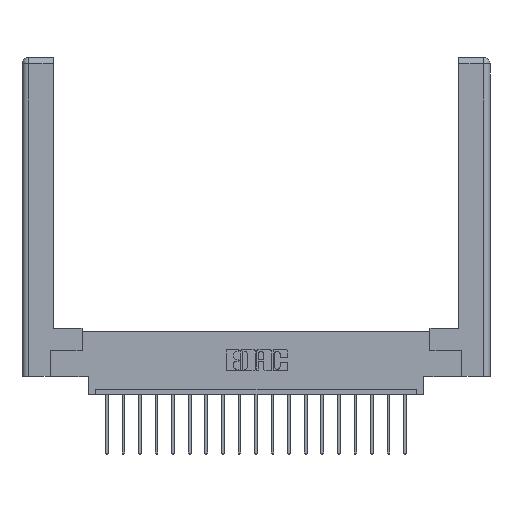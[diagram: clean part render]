
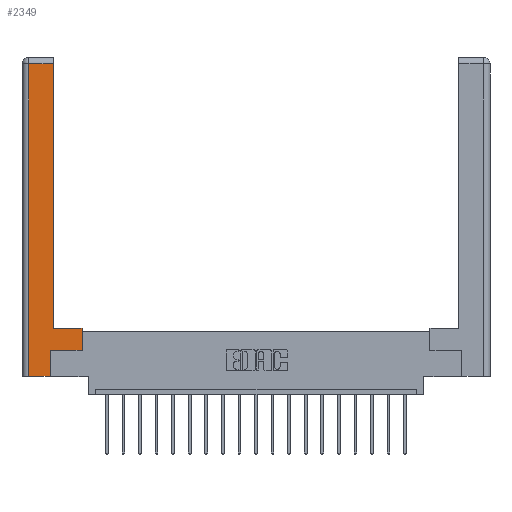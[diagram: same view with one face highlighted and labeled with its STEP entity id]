
A CAD part, top view. The second image highlights one B-rep face of the part: STEP entity #2349.
In plain terms, the highlighted planar face has unit normal (0, 0, 1).
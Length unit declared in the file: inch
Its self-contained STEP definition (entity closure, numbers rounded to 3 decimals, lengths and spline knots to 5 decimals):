
#362 = EDGE_CURVE ( 'NONE', #16933, #14075, #15181, .T. ) ;
#388 = EDGE_CURVE ( 'NONE', #4159, #2547, #11128, .T. ) ;
#723 = EDGE_CURVE ( 'NONE', #13145, #14437, #3665, .T. ) ;
#1186 = LINE ( 'NONE', #17285, #5532 ) ;
#1622 = CARTESIAN_POINT ( 'NONE',  ( 0.565, 0.245, 0. ) ) ;
#2067 = ORIENTED_EDGE ( 'NONE', *, *, #10837, .T. ) ;
#2349 = ADVANCED_FACE ( 'NONE', ( #7881 ), #5505, .F. ) ;
#2424 = VERTEX_POINT ( 'NONE', #3935 ) ;
#2462 = LINE ( 'NONE', #14794, #9640 ) ;
#2547 = VERTEX_POINT ( 'NONE', #1622 ) ;
#3395 = ORIENTED_EDGE ( 'NONE', *, *, #723, .T. ) ;
#3430 = DIRECTION ( 'NONE',  ( 1., 0., 0. ) ) ;
#3432 = VECTOR ( 'NONE', #10427, 39.37008 ) ;
#3541 = DIRECTION ( 'NONE',  ( 0., -1., 0. ) ) ;
#3665 = LINE ( 'NONE', #10676, #6324 ) ;
#3935 = CARTESIAN_POINT ( 'NONE',  ( 0.565, 0.45, 0. ) ) ;
#3956 = ORIENTED_EDGE ( 'NONE', *, *, #388, .T. ) ;
#4159 = VERTEX_POINT ( 'NONE', #4617 ) ;
#4617 = CARTESIAN_POINT ( 'NONE',  ( 0.265, 0.245, 0. ) ) ;
#5131 = DIRECTION ( 'NONE',  ( 1., 0., 0. ) ) ;
#5505 = PLANE ( 'NONE',  #16277 ) ;
#5532 = VECTOR ( 'NONE', #3430, 39.37008 ) ;
#5802 = LINE ( 'NONE', #10413, #13970 ) ;
#6008 = ORIENTED_EDGE ( 'NONE', *, *, #11953, .T. ) ;
#6324 = VECTOR ( 'NONE', #3541, 39.37008 ) ;
#6452 = LINE ( 'NONE', #17853, #6679 ) ;
#6679 = VECTOR ( 'NONE', #18226, 39.37008 ) ;
#6786 = CARTESIAN_POINT ( 'NONE',  ( 0.0615, 0., 0. ) ) ;
#7219 = DIRECTION ( 'NONE',  ( 0., 1., 0. ) ) ;
#7834 = EDGE_LOOP ( 'NONE', ( #15627, #13784, #3395, #6008, #15036, #3956, #2067, #12149 ) ) ;
#7881 = FACE_OUTER_BOUND ( 'NONE', #7834, .T. ) ;
#8752 = EDGE_CURVE ( 'NONE', #2424, #16933, #12839, .T. ) ;
#8883 = VERTEX_POINT ( 'NONE', #18029 ) ;
#9640 = VECTOR ( 'NONE', #7219, 39.37008 ) ;
#9772 = DIRECTION ( 'NONE',  ( -1., 0., 0. ) ) ;
#10413 = CARTESIAN_POINT ( 'NONE',  ( 0.265, 0.245, 0. ) ) ;
#10427 = DIRECTION ( 'NONE',  ( 0., 1., 0. ) ) ;
#10676 = CARTESIAN_POINT ( 'NONE',  ( 0.0615, 0., 0. ) ) ;
#10837 = EDGE_CURVE ( 'NONE', #2547, #2424, #2462, .T. ) ;
#11128 = LINE ( 'NONE', #18882, #19064 ) ;
#11131 = EDGE_CURVE ( 'NONE', #8883, #4159, #5802, .T. ) ;
#11900 = CARTESIAN_POINT ( 'NONE',  ( 0.0615, 2.94, 0. ) ) ;
#11953 = EDGE_CURVE ( 'NONE', #14437, #8883, #1186, .T. ) ;
#12149 = ORIENTED_EDGE ( 'NONE', *, *, #8752, .T. ) ;
#12839 = LINE ( 'NONE', #17646, #18861 ) ;
#12863 = DIRECTION ( 'NONE',  ( 0., 0., -1. ) ) ;
#13145 = VERTEX_POINT ( 'NONE', #11900 ) ;
#13166 = EDGE_CURVE ( 'NONE', #14075, #13145, #6452, .T. ) ;
#13564 = CARTESIAN_POINT ( 'NONE',  ( 0.295, 2.94, 0. ) ) ;
#13784 = ORIENTED_EDGE ( 'NONE', *, *, #13166, .T. ) ;
#13970 = VECTOR ( 'NONE', #16318, 39.37008 ) ;
#14075 = VERTEX_POINT ( 'NONE', #13564 ) ;
#14433 = CARTESIAN_POINT ( 'NONE',  ( 0.295, 0.45, 0. ) ) ;
#14437 = VERTEX_POINT ( 'NONE', #6786 ) ;
#14794 = CARTESIAN_POINT ( 'NONE',  ( 0.565, 0.45, 0. ) ) ;
#15036 = ORIENTED_EDGE ( 'NONE', *, *, #11131, .T. ) ;
#15181 = LINE ( 'NONE', #19615, #3432 ) ;
#15627 = ORIENTED_EDGE ( 'NONE', *, *, #362, .T. ) ;
#16229 = CARTESIAN_POINT ( 'NONE',  ( 0., 0., 0. ) ) ;
#16277 = AXIS2_PLACEMENT_3D ( 'NONE', #16229, #12863, #17533 ) ;
#16318 = DIRECTION ( 'NONE',  ( 0., 1., 0. ) ) ;
#16933 = VERTEX_POINT ( 'NONE', #14433 ) ;
#17285 = CARTESIAN_POINT ( 'NONE',  ( 0.265, 0., 0. ) ) ;
#17533 = DIRECTION ( 'NONE',  ( -1., 0., 0. ) ) ;
#17646 = CARTESIAN_POINT ( 'NONE',  ( 0.295, 0.45, 0. ) ) ;
#17853 = CARTESIAN_POINT ( 'NONE',  ( 0.0615, 2.94, 0. ) ) ;
#18029 = CARTESIAN_POINT ( 'NONE',  ( 0.265, 0., 0. ) ) ;
#18226 = DIRECTION ( 'NONE',  ( -1., 0., 0. ) ) ;
#18861 = VECTOR ( 'NONE', #9772, 39.37008 ) ;
#18882 = CARTESIAN_POINT ( 'NONE',  ( 0.565, 0.245, 0. ) ) ;
#19064 = VECTOR ( 'NONE', #5131, 39.37008 ) ;
#19615 = CARTESIAN_POINT ( 'NONE',  ( 0.295, 3., 0. ) ) ;
